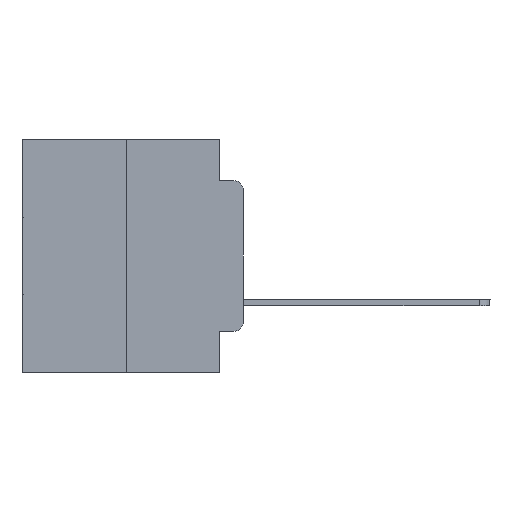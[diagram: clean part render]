
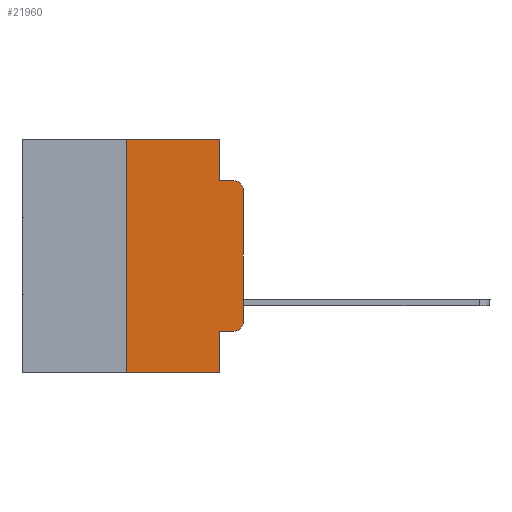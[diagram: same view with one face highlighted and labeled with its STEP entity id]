
A CAD part, left-side view. The second image highlights one B-rep face of the part: STEP entity #21960.
In plain terms, the highlighted planar face has unit normal (-1, 0, 0).
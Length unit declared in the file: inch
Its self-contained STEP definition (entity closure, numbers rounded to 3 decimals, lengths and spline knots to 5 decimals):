
#34 = ORIENTED_EDGE ( 'NONE', *, *, #11930, .F. ) ;
#117 = DIRECTION ( 'NONE',  ( 0., 0., -1. ) ) ;
#151 = VERTEX_POINT ( 'NONE', #24679 ) ;
#163 = EDGE_CURVE ( 'NONE', #3911, #7125, #24666, .T. ) ;
#268 = CIRCLE ( 'NONE', #4681, 0.02 ) ;
#1048 = VERTEX_POINT ( 'NONE', #4646 ) ;
#1503 = EDGE_CURVE ( 'NONE', #9064, #26330, #6538, .T. ) ;
#1721 = CARTESIAN_POINT ( 'NONE',  ( 0., 0., -0.3915 ) ) ;
#1726 = EDGE_CURVE ( 'NONE', #6958, #7125, #14120, .T. ) ;
#1822 = ORIENTED_EDGE ( 'NONE', *, *, #5536, .F. ) ;
#1916 = CARTESIAN_POINT ( 'NONE',  ( 0., 0.473, 0. ) ) ;
#3225 = LINE ( 'NONE', #12051, #11753 ) ;
#3548 = VECTOR ( 'NONE', #4474, 39.37008 ) ;
#3675 = VECTOR ( 'NONE', #10320, 39.37008 ) ;
#3911 = VERTEX_POINT ( 'NONE', #11404 ) ;
#4110 = FACE_OUTER_BOUND ( 'NONE', #24755, .T. ) ;
#4122 = VERTEX_POINT ( 'NONE', #10406 ) ;
#4474 = DIRECTION ( 'NONE',  ( 0., -1., 0. ) ) ;
#4646 = CARTESIAN_POINT ( 'NONE',  ( 0., 0.25, -0.5 ) ) ;
#4669 = ORIENTED_EDGE ( 'NONE', *, *, #1726, .F. ) ;
#4681 = AXIS2_PLACEMENT_3D ( 'NONE', #6485, #6345, #10629 ) ;
#4932 = VECTOR ( 'NONE', #19150, 39.37008 ) ;
#5382 = CARTESIAN_POINT ( 'NONE',  ( 0., 0.051, 0. ) ) ;
#5536 = EDGE_CURVE ( 'NONE', #4122, #151, #3225, .T. ) ;
#5544 = DIRECTION ( 'NONE',  ( 0., -1., 0. ) ) ;
#5758 = CARTESIAN_POINT ( 'NONE',  ( 0., 0.051, -0.4115 ) ) ;
#5978 = DIRECTION ( 'NONE',  ( -1., 0., 0. ) ) ;
#6345 = DIRECTION ( 'NONE',  ( -1., 0., 0. ) ) ;
#6485 = CARTESIAN_POINT ( 'NONE',  ( 0., 0.02, -0.3915 ) ) ;
#6538 = LINE ( 'NONE', #23303, #3548 ) ;
#6618 = EDGE_CURVE ( 'NONE', #1048, #4122, #8516, .T. ) ;
#6874 = LINE ( 'NONE', #13222, #25067 ) ;
#6958 = VERTEX_POINT ( 'NONE', #17126 ) ;
#7125 = VERTEX_POINT ( 'NONE', #24081 ) ;
#7290 = ORIENTED_EDGE ( 'NONE', *, *, #6618, .F. ) ;
#7955 = LINE ( 'NONE', #14315, #23190 ) ;
#8065 = CARTESIAN_POINT ( 'NONE',  ( 0., 0.02, -0.1085 ) ) ;
#8516 = LINE ( 'NONE', #14464, #23173 ) ;
#9064 = VERTEX_POINT ( 'NONE', #5758 ) ;
#10166 = ORIENTED_EDGE ( 'NONE', *, *, #25878, .T. ) ;
#10320 = DIRECTION ( 'NONE',  ( 0., 0., -1. ) ) ;
#10406 = CARTESIAN_POINT ( 'NONE',  ( 0., 0.25, 0. ) ) ;
#10463 = DIRECTION ( 'NONE',  ( 0., -1., 0. ) ) ;
#10597 = PLANE ( 'NONE',  #15188 ) ;
#10629 = DIRECTION ( 'NONE',  ( 0., 0., -1. ) ) ;
#11389 = EDGE_CURVE ( 'NONE', #1048, #18881, #6874, .T. ) ;
#11404 = CARTESIAN_POINT ( 'NONE',  ( 0., 0., -0.1085 ) ) ;
#11432 = ORIENTED_EDGE ( 'NONE', *, *, #163, .T. ) ;
#11753 = VECTOR ( 'NONE', #20392, 39.37008 ) ;
#11930 = EDGE_CURVE ( 'NONE', #151, #6958, #17247, .T. ) ;
#12051 = CARTESIAN_POINT ( 'NONE',  ( 0., 0.473, 0. ) ) ;
#12111 = DIRECTION ( 'NONE',  ( 0., 0., 1. ) ) ;
#13043 = VERTEX_POINT ( 'NONE', #1721 ) ;
#13222 = CARTESIAN_POINT ( 'NONE',  ( 0., 0.473, -0.5 ) ) ;
#13763 = AXIS2_PLACEMENT_3D ( 'NONE', #8065, #5978, #26596 ) ;
#14120 = LINE ( 'NONE', #20387, #22069 ) ;
#14315 = CARTESIAN_POINT ( 'NONE',  ( 0., 0., 0. ) ) ;
#14464 = CARTESIAN_POINT ( 'NONE',  ( 0., 0.25, 0. ) ) ;
#15188 = AXIS2_PLACEMENT_3D ( 'NONE', #1916, #18976, #117 ) ;
#16273 = ORIENTED_EDGE ( 'NONE', *, *, #1503, .T. ) ;
#16530 = LINE ( 'NONE', #5382, #3675 ) ;
#17126 = CARTESIAN_POINT ( 'NONE',  ( 0., 0.051, -0.0885 ) ) ;
#17247 = LINE ( 'NONE', #25313, #4932 ) ;
#18881 = VERTEX_POINT ( 'NONE', #18966 ) ;
#18966 = CARTESIAN_POINT ( 'NONE',  ( 0., 0.051, -0.5 ) ) ;
#18976 = DIRECTION ( 'NONE',  ( 1., 0., 0. ) ) ;
#19150 = DIRECTION ( 'NONE',  ( 0., 0., -1. ) ) ;
#19735 = ORIENTED_EDGE ( 'NONE', *, *, #11389, .T. ) ;
#19998 = EDGE_CURVE ( 'NONE', #9064, #18881, #16530, .T. ) ;
#20146 = CARTESIAN_POINT ( 'NONE',  ( 0., 0.02, -0.4115 ) ) ;
#20387 = CARTESIAN_POINT ( 'NONE',  ( 0., 0.051, -0.0885 ) ) ;
#20392 = DIRECTION ( 'NONE',  ( 0., -1., 0. ) ) ;
#21960 = ADVANCED_FACE ( 'NONE', ( #4110 ), #10597, .F. ) ;
#22069 = VECTOR ( 'NONE', #5544, 39.37008 ) ;
#23173 = VECTOR ( 'NONE', #27048, 39.37008 ) ;
#23190 = VECTOR ( 'NONE', #12111, 39.37008 ) ;
#23303 = CARTESIAN_POINT ( 'NONE',  ( 0., 0.051, -0.4115 ) ) ;
#23401 = ORIENTED_EDGE ( 'NONE', *, *, #19998, .F. ) ;
#24002 = EDGE_CURVE ( 'NONE', #26330, #13043, #268, .T. ) ;
#24081 = CARTESIAN_POINT ( 'NONE',  ( 0., 0.02, -0.0885 ) ) ;
#24446 = ORIENTED_EDGE ( 'NONE', *, *, #24002, .T. ) ;
#24666 = CIRCLE ( 'NONE', #13763, 0.02 ) ;
#24679 = CARTESIAN_POINT ( 'NONE',  ( 0., 0.051, 0. ) ) ;
#24755 = EDGE_LOOP ( 'NONE', ( #10166, #11432, #4669, #34, #1822, #7290, #19735, #23401, #16273, #24446 ) ) ;
#25067 = VECTOR ( 'NONE', #10463, 39.37008 ) ;
#25313 = CARTESIAN_POINT ( 'NONE',  ( 0., 0.051, 0. ) ) ;
#25878 = EDGE_CURVE ( 'NONE', #13043, #3911, #7955, .T. ) ;
#26330 = VERTEX_POINT ( 'NONE', #20146 ) ;
#26596 = DIRECTION ( 'NONE',  ( 0., 0., -1. ) ) ;
#27048 = DIRECTION ( 'NONE',  ( 0., 0., 1. ) ) ;
